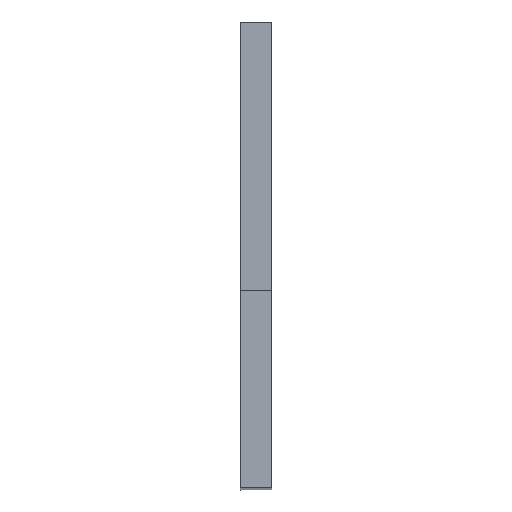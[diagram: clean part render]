
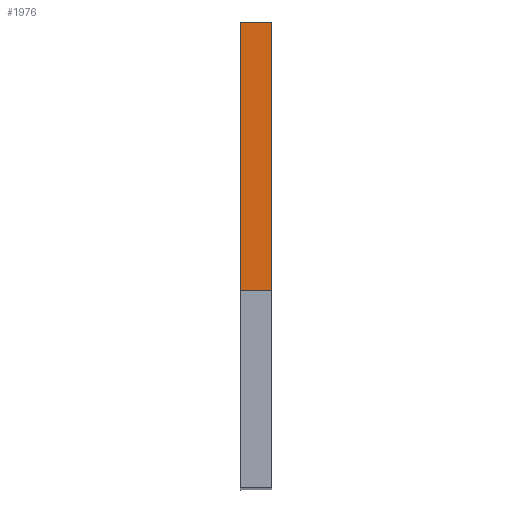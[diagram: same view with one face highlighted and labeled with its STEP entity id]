
A CAD part, top view. The second image highlights one B-rep face of the part: STEP entity #1976.
In plain terms, the highlighted planar face has unit normal (0, 0, 1).
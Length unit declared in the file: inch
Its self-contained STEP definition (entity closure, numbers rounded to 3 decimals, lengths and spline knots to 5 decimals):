
#66=PLANE('',#2121);
#168=FACE_OUTER_BOUND('',#296,.T.);
#296=EDGE_LOOP('',(#1793,#1794,#1795,#1796));
#572=LINE('',#4289,#670);
#574=LINE('',#4293,#672);
#588=LINE('',#5367,#686);
#598=LINE('',#7540,#696);
#670=VECTOR('',#2382,0.3937);
#672=VECTOR('',#2386,0.3937);
#686=VECTOR('',#2416,0.3937);
#696=VECTOR('',#2480,0.3937);
#870=VERTEX_POINT('',#4286);
#871=VERTEX_POINT('',#4288);
#872=VERTEX_POINT('',#4292);
#891=VERTEX_POINT('',#5365);
#1108=EDGE_CURVE('',#870,#871,#572,.T.);
#1110=EDGE_CURVE('',#871,#872,#574,.T.);
#1152=EDGE_CURVE('',#891,#870,#588,.T.);
#1198=EDGE_CURVE('',#891,#872,#598,.T.);
#1793=ORIENTED_EDGE('',*,*,#1152,.F.);
#1794=ORIENTED_EDGE('',*,*,#1198,.T.);
#1795=ORIENTED_EDGE('',*,*,#1110,.F.);
#1796=ORIENTED_EDGE('',*,*,#1108,.F.);
#1976=ADVANCED_FACE('',(#168),#66,.T.);
#2121=AXIS2_PLACEMENT_3D('',#7541,#2481,#2482);
#2382=DIRECTION('',(1.,0.,0.));
#2386=DIRECTION('',(0.,-1.,0.));
#2416=DIRECTION('',(0.,1.,0.));
#2480=DIRECTION('',(1.,0.,0.));
#2481=DIRECTION('center_axis',(0.,0.,1.));
#2482=DIRECTION('ref_axis',(0.,-1.,0.));
#4286=CARTESIAN_POINT('',(0.363,0.,0.285));
#4288=CARTESIAN_POINT('',(0.453,0.,0.285));
#4289=CARTESIAN_POINT('',(0.363,0.,0.285));
#4292=CARTESIAN_POINT('',(0.453,-0.768,0.285));
#4293=CARTESIAN_POINT('',(0.453,-0.33375,0.285));
#5365=CARTESIAN_POINT('',(0.363,-0.768,0.285));
#5367=CARTESIAN_POINT('',(0.363,-0.33375,0.285));
#7540=CARTESIAN_POINT('',(0.363,-0.768,0.285));
#7541=CARTESIAN_POINT('Origin',(0.363,0.,0.285));
